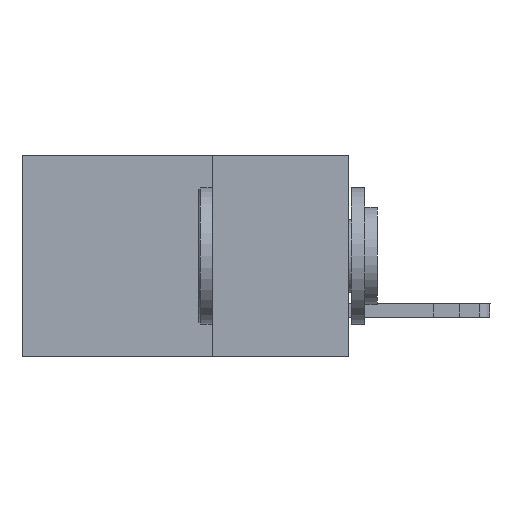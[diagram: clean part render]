
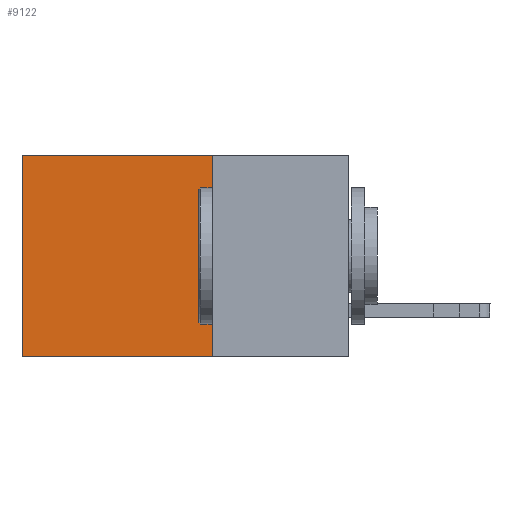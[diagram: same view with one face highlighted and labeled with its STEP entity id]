
A CAD part, left-side view. The second image highlights one B-rep face of the part: STEP entity #9122.
In plain terms, the highlighted planar face has unit normal (-1, 0, 0).
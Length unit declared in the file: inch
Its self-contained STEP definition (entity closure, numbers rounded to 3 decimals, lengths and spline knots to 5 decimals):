
#621 = PLANE ( 'NONE',  #12047 ) ;
#787 = VECTOR ( 'NONE', #11176, 39.37008 ) ;
#934 = DIRECTION ( 'NONE',  ( 0., 0., -1. ) ) ;
#1677 = CARTESIAN_POINT ( 'NONE',  ( 0.298, 0.6, -0.37 ) ) ;
#1691 = LINE ( 'NONE', #3091, #787 ) ;
#1783 = FACE_OUTER_BOUND ( 'NONE', #4822, .T. ) ;
#2129 = ORIENTED_EDGE ( 'NONE', *, *, #14253, .T. ) ;
#2321 = VERTEX_POINT ( 'NONE', #12818 ) ;
#2588 = VERTEX_POINT ( 'NONE', #1677 ) ;
#3086 = CARTESIAN_POINT ( 'NONE',  ( 0.298, 0.25, 0. ) ) ;
#3091 = CARTESIAN_POINT ( 'NONE',  ( 0.298, 0.25, 0. ) ) ;
#3395 = LINE ( 'NONE', #11497, #7023 ) ;
#3894 = LINE ( 'NONE', #6048, #8092 ) ;
#3911 = EDGE_CURVE ( 'NONE', #2321, #2588, #12308, .T. ) ;
#4072 = DIRECTION ( 'NONE',  ( 0., 1., 0. ) ) ;
#4115 = VECTOR ( 'NONE', #4072, 39.37008 ) ;
#4619 = ORIENTED_EDGE ( 'NONE', *, *, #11079, .F. ) ;
#4822 = EDGE_LOOP ( 'NONE', ( #2129, #12180, #4619, #7586 ) ) ;
#6048 = CARTESIAN_POINT ( 'NONE',  ( 0.298, 0.25, 0. ) ) ;
#6946 = EDGE_CURVE ( 'NONE', #10804, #7130, #3894, .T. ) ;
#7023 = VECTOR ( 'NONE', #934, 39.37008 ) ;
#7130 = VERTEX_POINT ( 'NONE', #11458 ) ;
#7586 = ORIENTED_EDGE ( 'NONE', *, *, #6946, .T. ) ;
#7631 = DIRECTION ( 'NONE',  ( 1., 0., 0. ) ) ;
#8092 = VECTOR ( 'NONE', #14293, 39.37008 ) ;
#8706 = CARTESIAN_POINT ( 'NONE',  ( 0.298, 0.25, 0. ) ) ;
#9122 = ADVANCED_FACE ( 'NONE', ( #1783 ), #621, .F. ) ;
#10804 = VERTEX_POINT ( 'NONE', #3086 ) ;
#11079 = EDGE_CURVE ( 'NONE', #10804, #2321, #1691, .T. ) ;
#11176 = DIRECTION ( 'NONE',  ( 0., 0., -1. ) ) ;
#11458 = CARTESIAN_POINT ( 'NONE',  ( 0.298, 0.6, 0. ) ) ;
#11497 = CARTESIAN_POINT ( 'NONE',  ( 0.298, 0.6, 0. ) ) ;
#12047 = AXIS2_PLACEMENT_3D ( 'NONE', #8706, #7631, #13416 ) ;
#12180 = ORIENTED_EDGE ( 'NONE', *, *, #3911, .F. ) ;
#12308 = LINE ( 'NONE', #14706, #4115 ) ;
#12818 = CARTESIAN_POINT ( 'NONE',  ( 0.298, 0.25, -0.37 ) ) ;
#13416 = DIRECTION ( 'NONE',  ( 0., 0., -1. ) ) ;
#14253 = EDGE_CURVE ( 'NONE', #7130, #2588, #3395, .T. ) ;
#14293 = DIRECTION ( 'NONE',  ( 0., 1., 0. ) ) ;
#14706 = CARTESIAN_POINT ( 'NONE',  ( 0.298, 0.25, -0.37 ) ) ;
